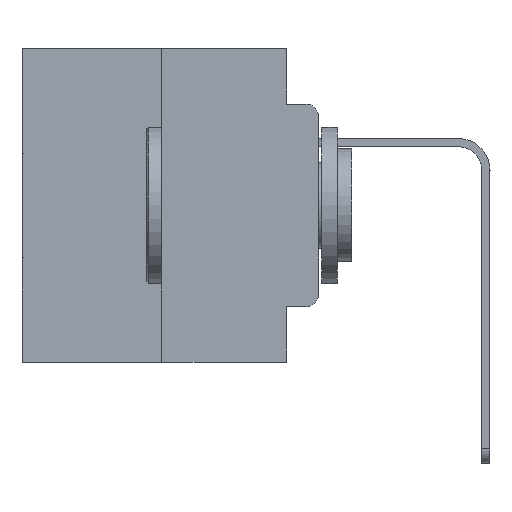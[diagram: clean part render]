
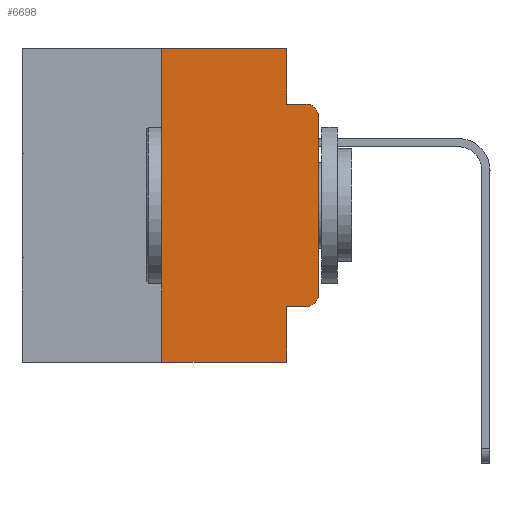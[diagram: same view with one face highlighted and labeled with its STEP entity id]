
A CAD part, left-side view. The second image highlights one B-rep face of the part: STEP entity #6698.
In plain terms, the highlighted planar face has unit normal (-1, 0, 0).
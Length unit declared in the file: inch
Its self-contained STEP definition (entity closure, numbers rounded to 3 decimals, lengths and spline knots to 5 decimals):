
#186 = EDGE_LOOP ( 'NONE', ( #6222, #1456, #20937, #2147, #19477, #15697, #16349, #15112, #23424, #19582 ) ) ;
#299 = CARTESIAN_POINT ( 'NONE',  ( 0., 0.02, -0.0885 ) ) ;
#313 = DIRECTION ( 'NONE',  ( 0., 0., -1. ) ) ;
#610 = EDGE_CURVE ( 'NONE', #24929, #6120, #10537, .T. ) ;
#835 = LINE ( 'NONE', #23655, #9591 ) ;
#1029 = LINE ( 'NONE', #24539, #25715 ) ;
#1155 = DIRECTION ( 'NONE',  ( 0., -1., 0. ) ) ;
#1189 = VERTEX_POINT ( 'NONE', #4261 ) ;
#1456 = ORIENTED_EDGE ( 'NONE', *, *, #610, .T. ) ;
#2025 = CIRCLE ( 'NONE', #8555, 0.02 ) ;
#2147 = ORIENTED_EDGE ( 'NONE', *, *, #6820, .F. ) ;
#2353 = DIRECTION ( 'NONE',  ( -1., 0., 0. ) ) ;
#2490 = LINE ( 'NONE', #23457, #23886 ) ;
#2970 = CARTESIAN_POINT ( 'NONE',  ( 0., 0.051, 0. ) ) ;
#3780 = AXIS2_PLACEMENT_3D ( 'NONE', #13388, #15520, #17664 ) ;
#4111 = AXIS2_PLACEMENT_3D ( 'NONE', #23849, #2353, #313 ) ;
#4258 = EDGE_CURVE ( 'NONE', #7986, #19098, #26865, .T. ) ;
#4261 = CARTESIAN_POINT ( 'NONE',  ( 0., 0.051, -0.0885 ) ) ;
#4456 = EDGE_CURVE ( 'NONE', #26159, #19098, #8219, .T. ) ;
#5108 = CARTESIAN_POINT ( 'NONE',  ( 0., 0.25, -0.5 ) ) ;
#5808 = VERTEX_POINT ( 'NONE', #16129 ) ;
#6120 = VERTEX_POINT ( 'NONE', #299 ) ;
#6222 = ORIENTED_EDGE ( 'NONE', *, *, #25517, .T. ) ;
#6698 = ADVANCED_FACE ( 'NONE', ( #18747 ), #6918, .F. ) ;
#6820 = EDGE_CURVE ( 'NONE', #23224, #1189, #19760, .T. ) ;
#6918 = PLANE ( 'NONE',  #3780 ) ;
#7215 = LINE ( 'NONE', #11858, #11272 ) ;
#7986 = VERTEX_POINT ( 'NONE', #18642 ) ;
#8219 = LINE ( 'NONE', #20531, #9585 ) ;
#8555 = AXIS2_PLACEMENT_3D ( 'NONE', #27298, #18780, #14509 ) ;
#9585 = VECTOR ( 'NONE', #26892, 39.37008 ) ;
#9591 = VECTOR ( 'NONE', #17230, 39.37008 ) ;
#9676 = DIRECTION ( 'NONE',  ( 0., 0., 1. ) ) ;
#10537 = CIRCLE ( 'NONE', #4111, 0.02 ) ;
#11240 = CARTESIAN_POINT ( 'NONE',  ( 0., 0.02, -0.4115 ) ) ;
#11272 = VECTOR ( 'NONE', #1155, 39.37008 ) ;
#11327 = DIRECTION ( 'NONE',  ( 0., 0., -1. ) ) ;
#11858 = CARTESIAN_POINT ( 'NONE',  ( 0., 0.473, 0. ) ) ;
#12483 = EDGE_CURVE ( 'NONE', #7986, #19060, #18623, .T. ) ;
#13388 = CARTESIAN_POINT ( 'NONE',  ( 0., 0.473, 0. ) ) ;
#13940 = EDGE_CURVE ( 'NONE', #26000, #23224, #7215, .T. ) ;
#14260 = EDGE_CURVE ( 'NONE', #1189, #6120, #2490, .T. ) ;
#14509 = DIRECTION ( 'NONE',  ( 0., 0., -1. ) ) ;
#14895 = DIRECTION ( 'NONE',  ( 0., -1., 0. ) ) ;
#15112 = ORIENTED_EDGE ( 'NONE', *, *, #4258, .F. ) ;
#15311 = CARTESIAN_POINT ( 'NONE',  ( 0., 0.25, 0. ) ) ;
#15322 = CARTESIAN_POINT ( 'NONE',  ( 0., 0., -0.1085 ) ) ;
#15520 = DIRECTION ( 'NONE',  ( 1., 0., 0. ) ) ;
#15697 = ORIENTED_EDGE ( 'NONE', *, *, #19562, .F. ) ;
#15949 = VECTOR ( 'NONE', #22186, 39.37008 ) ;
#16129 = CARTESIAN_POINT ( 'NONE',  ( 0., 0., -0.3915 ) ) ;
#16349 = ORIENTED_EDGE ( 'NONE', *, *, #4456, .T. ) ;
#17230 = DIRECTION ( 'NONE',  ( 0., 0., 1. ) ) ;
#17664 = DIRECTION ( 'NONE',  ( 0., 0., -1. ) ) ;
#18623 = LINE ( 'NONE', #22093, #15949 ) ;
#18642 = CARTESIAN_POINT ( 'NONE',  ( 0., 0.051, -0.4115 ) ) ;
#18747 = FACE_OUTER_BOUND ( 'NONE', #186, .T. ) ;
#18780 = DIRECTION ( 'NONE',  ( -1., 0., 0. ) ) ;
#19060 = VERTEX_POINT ( 'NONE', #11240 ) ;
#19078 = VECTOR ( 'NONE', #24346, 39.37008 ) ;
#19098 = VERTEX_POINT ( 'NONE', #21938 ) ;
#19477 = ORIENTED_EDGE ( 'NONE', *, *, #13940, .F. ) ;
#19562 = EDGE_CURVE ( 'NONE', #26159, #26000, #835, .T. ) ;
#19582 = ORIENTED_EDGE ( 'NONE', *, *, #25250, .T. ) ;
#19760 = LINE ( 'NONE', #2970, #19078 ) ;
#20531 = CARTESIAN_POINT ( 'NONE',  ( 0., 0.473, -0.5 ) ) ;
#20937 = ORIENTED_EDGE ( 'NONE', *, *, #14260, .F. ) ;
#21931 = CARTESIAN_POINT ( 'NONE',  ( 0., 0.051, 0. ) ) ;
#21938 = CARTESIAN_POINT ( 'NONE',  ( 0., 0.051, -0.5 ) ) ;
#22093 = CARTESIAN_POINT ( 'NONE',  ( 0., 0.051, -0.4115 ) ) ;
#22186 = DIRECTION ( 'NONE',  ( 0., -1., 0. ) ) ;
#23224 = VERTEX_POINT ( 'NONE', #24623 ) ;
#23424 = ORIENTED_EDGE ( 'NONE', *, *, #12483, .T. ) ;
#23457 = CARTESIAN_POINT ( 'NONE',  ( 0., 0.051, -0.0885 ) ) ;
#23655 = CARTESIAN_POINT ( 'NONE',  ( 0., 0.25, 0. ) ) ;
#23849 = CARTESIAN_POINT ( 'NONE',  ( 0., 0.02, -0.1085 ) ) ;
#23886 = VECTOR ( 'NONE', #14895, 39.37008 ) ;
#24346 = DIRECTION ( 'NONE',  ( 0., 0., -1. ) ) ;
#24539 = CARTESIAN_POINT ( 'NONE',  ( 0., 0., 0. ) ) ;
#24623 = CARTESIAN_POINT ( 'NONE',  ( 0., 0.051, 0. ) ) ;
#24929 = VERTEX_POINT ( 'NONE', #15322 ) ;
#25250 = EDGE_CURVE ( 'NONE', #19060, #5808, #2025, .T. ) ;
#25517 = EDGE_CURVE ( 'NONE', #5808, #24929, #1029, .T. ) ;
#25715 = VECTOR ( 'NONE', #9676, 39.37008 ) ;
#26000 = VERTEX_POINT ( 'NONE', #15311 ) ;
#26159 = VERTEX_POINT ( 'NONE', #5108 ) ;
#26539 = VECTOR ( 'NONE', #11327, 39.37008 ) ;
#26865 = LINE ( 'NONE', #21931, #26539 ) ;
#26892 = DIRECTION ( 'NONE',  ( 0., -1., 0. ) ) ;
#27298 = CARTESIAN_POINT ( 'NONE',  ( 0., 0.02, -0.3915 ) ) ;
